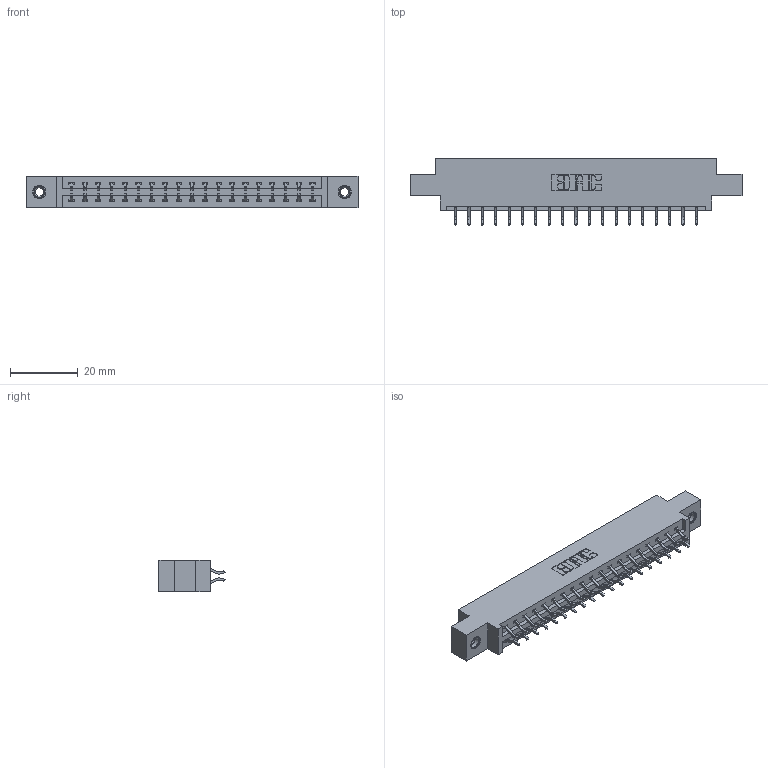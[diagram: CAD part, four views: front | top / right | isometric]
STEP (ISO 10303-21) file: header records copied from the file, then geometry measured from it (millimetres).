
FILE_DESCRIPTION (( 'STEP AP203' ), '1' );
FILE_NAME ('337-038-556-807.STEP', '2018-08-08T05:31:45', ( '' ), ( '' ), 'SwSTEP 2.0', 'SolidWorks 2016', '' );
FILE_SCHEMA (( 'CONFIG_CONTROL_DESIGN' ));
Length unit declared in the file: inch
Products named in the file (4): 337 Part_0.170 Offset - 0.156 Dia-TI; 345-292-001_556 Tail; 345-250-001_345-250-005-103; 337-038-556-807
Assembly tree (41 placements, depth 2):
  337-038-556-807
    337 Part_0.170 Offset - 0.156 Dia-TI
    345-292-001_556 Tail  x38
    345-250-001_345-250-005-103  x2
Bounding box: 98.3 x 19.57 x 9.4 mm (x, y, z)
Volume: 9920.7 mm3; surface area: 11095.7 mm2
Topology: 41 solids, 41 shells, 2458 faces, 7261 edges, 4782 vertices
Faces by surface type: plane 1702, cylinder 740, cone 12, torus 4
Entity records: 19244 total; most frequent: CARTESIAN_POINT 3257, ORIENTED_EDGE 3174, DIRECTION 2833, EDGE_CURVE 1587, LINE 1431, VECTOR 1431, VERTEX_POINT 1052, AXIS2_PLACEMENT_3D 701
